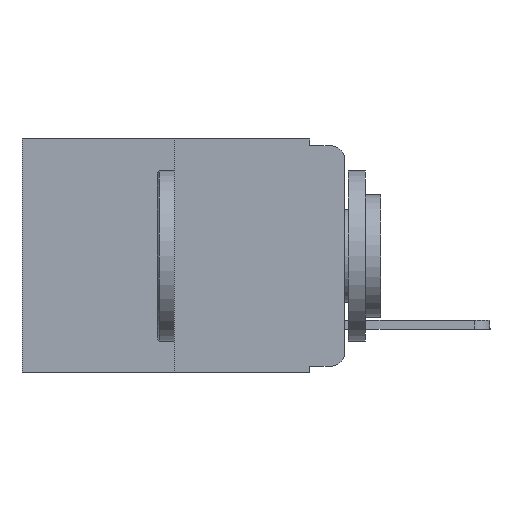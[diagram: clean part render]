
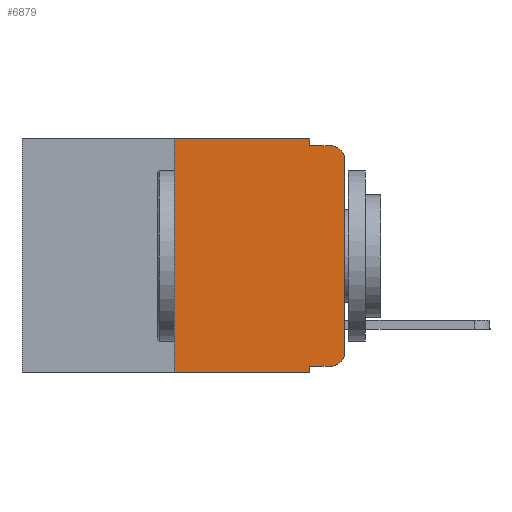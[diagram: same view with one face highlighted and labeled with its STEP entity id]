
A CAD part, left-side view. The second image highlights one B-rep face of the part: STEP entity #6879.
In plain terms, the highlighted planar face has unit normal (-1, 0, 0).
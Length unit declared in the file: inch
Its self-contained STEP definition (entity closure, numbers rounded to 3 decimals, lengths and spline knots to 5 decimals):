
#169 = ORIENTED_EDGE ( 'NONE', *, *, #7247, .F. ) ;
#216 = ORIENTED_EDGE ( 'NONE', *, *, #7668, .T. ) ;
#440 = VERTEX_POINT ( 'NONE', #11470 ) ;
#473 = CARTESIAN_POINT ( 'NONE',  ( 0., 0.473, -0.343 ) ) ;
#561 = VERTEX_POINT ( 'NONE', #662 ) ;
#592 = CARTESIAN_POINT ( 'NONE',  ( 0., 0.051, -0.01 ) ) ;
#662 = CARTESIAN_POINT ( 'NONE',  ( 0., 0., -0.313 ) ) ;
#961 = DIRECTION ( 'NONE',  ( 1., 0., 0. ) ) ;
#1084 = DIRECTION ( 'NONE',  ( 0., 0., 1. ) ) ;
#1285 = EDGE_LOOP ( 'NONE', ( #2574, #7870, #10269, #169, #8063, #7763, #5558, #3329, #216, #3343 ) ) ;
#1390 = LINE ( 'NONE', #7053, #5579 ) ;
#1490 = DIRECTION ( 'NONE',  ( 0., 0., -1. ) ) ;
#1582 = CIRCLE ( 'NONE', #3223, 0.02 ) ;
#1771 = LINE ( 'NONE', #8510, #4820 ) ;
#1828 = DIRECTION ( 'NONE',  ( -1., 0., 0. ) ) ;
#2011 = EDGE_CURVE ( 'NONE', #561, #9912, #1771, .T. ) ;
#2194 = VERTEX_POINT ( 'NONE', #4481 ) ;
#2239 = CARTESIAN_POINT ( 'NONE',  ( 0., 0.051, -0.333 ) ) ;
#2382 = CARTESIAN_POINT ( 'NONE',  ( 0., 0.051, 0. ) ) ;
#2520 = VECTOR ( 'NONE', #9862, 39.37008 ) ;
#2566 = PLANE ( 'NONE',  #10894 ) ;
#2574 = ORIENTED_EDGE ( 'NONE', *, *, #2011, .T. ) ;
#2682 = FACE_OUTER_BOUND ( 'NONE', #1285, .T. ) ;
#3223 = AXIS2_PLACEMENT_3D ( 'NONE', #7090, #6082, #1490 ) ;
#3310 = CARTESIAN_POINT ( 'NONE',  ( 0., 0.051, 0. ) ) ;
#3329 = ORIENTED_EDGE ( 'NONE', *, *, #4975, .F. ) ;
#3333 = VECTOR ( 'NONE', #5071, 39.37008 ) ;
#3343 = ORIENTED_EDGE ( 'NONE', *, *, #7638, .T. ) ;
#4025 = EDGE_CURVE ( 'NONE', #7652, #10121, #8864, .T. ) ;
#4162 = LINE ( 'NONE', #3310, #4612 ) ;
#4232 = EDGE_CURVE ( 'NONE', #10571, #2194, #1390, .T. ) ;
#4479 = VECTOR ( 'NONE', #4931, 39.37008 ) ;
#4481 = CARTESIAN_POINT ( 'NONE',  ( 0., 0.02, -0.01 ) ) ;
#4511 = DIRECTION ( 'NONE',  ( 0., 0., -1. ) ) ;
#4612 = VECTOR ( 'NONE', #6060, 39.37008 ) ;
#4780 = DIRECTION ( 'NONE',  ( 0., -1., 0. ) ) ;
#4820 = VECTOR ( 'NONE', #1084, 39.37008 ) ;
#4931 = DIRECTION ( 'NONE',  ( 0., -1., 0. ) ) ;
#4975 = EDGE_CURVE ( 'NONE', #11431, #10121, #4162, .T. ) ;
#5071 = DIRECTION ( 'NONE',  ( 0., 0., 1. ) ) ;
#5232 = VERTEX_POINT ( 'NONE', #7251 ) ;
#5493 = CARTESIAN_POINT ( 'NONE',  ( 0., 0., -0.03 ) ) ;
#5558 = ORIENTED_EDGE ( 'NONE', *, *, #4025, .T. ) ;
#5579 = VECTOR ( 'NONE', #8875, 39.37008 ) ;
#5619 = CARTESIAN_POINT ( 'NONE',  ( 0., 0.02, -0.03 ) ) ;
#5982 = CARTESIAN_POINT ( 'NONE',  ( 0., 0.051, -0.343 ) ) ;
#6060 = DIRECTION ( 'NONE',  ( 0., 0., -1. ) ) ;
#6082 = DIRECTION ( 'NONE',  ( -1., 0., 0. ) ) ;
#6159 = VECTOR ( 'NONE', #8000, 39.37008 ) ;
#6547 = AXIS2_PLACEMENT_3D ( 'NONE', #5619, #1828, #4511 ) ;
#6790 = CARTESIAN_POINT ( 'NONE',  ( 0., 0.473, 0. ) ) ;
#6809 = CARTESIAN_POINT ( 'NONE',  ( 0., 0.051, -0.333 ) ) ;
#6879 = ADVANCED_FACE ( 'NONE', ( #2682 ), #2566, .F. ) ;
#7053 = CARTESIAN_POINT ( 'NONE',  ( 0., 0.051, -0.01 ) ) ;
#7090 = CARTESIAN_POINT ( 'NONE',  ( 0., 0.02, -0.313 ) ) ;
#7247 = EDGE_CURVE ( 'NONE', #5232, #10571, #10783, .T. ) ;
#7251 = CARTESIAN_POINT ( 'NONE',  ( 0., 0.051, 0. ) ) ;
#7535 = CIRCLE ( 'NONE', #6547, 0.02 ) ;
#7638 = EDGE_CURVE ( 'NONE', #440, #561, #1582, .T. ) ;
#7652 = VERTEX_POINT ( 'NONE', #9844 ) ;
#7668 = EDGE_CURVE ( 'NONE', #11431, #440, #9903, .T. ) ;
#7763 = ORIENTED_EDGE ( 'NONE', *, *, #8486, .F. ) ;
#7870 = ORIENTED_EDGE ( 'NONE', *, *, #9928, .T. ) ;
#8000 = DIRECTION ( 'NONE',  ( 0., -1., 0. ) ) ;
#8063 = ORIENTED_EDGE ( 'NONE', *, *, #8807, .F. ) ;
#8260 = DIRECTION ( 'NONE',  ( 0., 0., -1. ) ) ;
#8486 = EDGE_CURVE ( 'NONE', #7652, #11482, #9058, .T. ) ;
#8510 = CARTESIAN_POINT ( 'NONE',  ( 0., 0., 0. ) ) ;
#8807 = EDGE_CURVE ( 'NONE', #11482, #5232, #9479, .T. ) ;
#8864 = LINE ( 'NONE', #473, #11476 ) ;
#8875 = DIRECTION ( 'NONE',  ( 0., -1., 0. ) ) ;
#9058 = LINE ( 'NONE', #11672, #3333 ) ;
#9479 = LINE ( 'NONE', #6790, #4479 ) ;
#9844 = CARTESIAN_POINT ( 'NONE',  ( 0., 0.25, -0.343 ) ) ;
#9862 = DIRECTION ( 'NONE',  ( 0., 0., -1. ) ) ;
#9903 = LINE ( 'NONE', #2239, #6159 ) ;
#9912 = VERTEX_POINT ( 'NONE', #5493 ) ;
#9928 = EDGE_CURVE ( 'NONE', #9912, #2194, #7535, .T. ) ;
#10121 = VERTEX_POINT ( 'NONE', #5982 ) ;
#10269 = ORIENTED_EDGE ( 'NONE', *, *, #4232, .F. ) ;
#10571 = VERTEX_POINT ( 'NONE', #592 ) ;
#10783 = LINE ( 'NONE', #2382, #2520 ) ;
#10894 = AXIS2_PLACEMENT_3D ( 'NONE', #11098, #961, #8260 ) ;
#11098 = CARTESIAN_POINT ( 'NONE',  ( 0., 0.473, 0. ) ) ;
#11431 = VERTEX_POINT ( 'NONE', #6809 ) ;
#11470 = CARTESIAN_POINT ( 'NONE',  ( 0., 0.02, -0.333 ) ) ;
#11476 = VECTOR ( 'NONE', #4780, 39.37008 ) ;
#11482 = VERTEX_POINT ( 'NONE', #11861 ) ;
#11672 = CARTESIAN_POINT ( 'NONE',  ( 0., 0.25, 0. ) ) ;
#11861 = CARTESIAN_POINT ( 'NONE',  ( 0., 0.25, 0. ) ) ;
